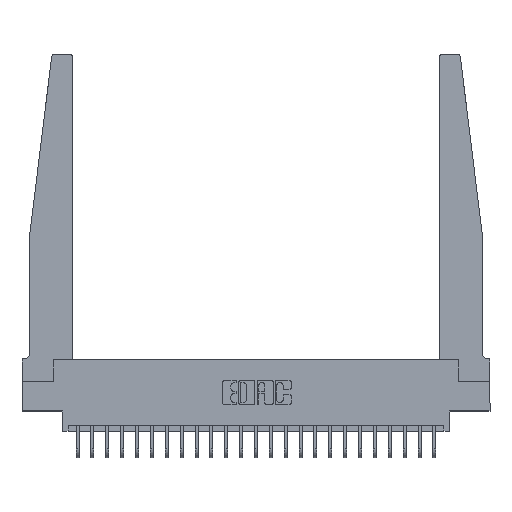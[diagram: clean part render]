
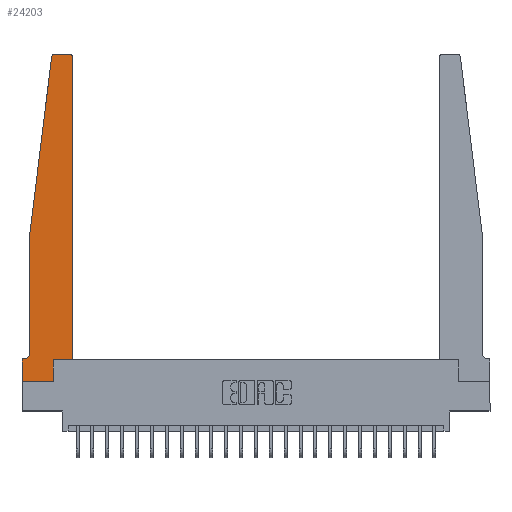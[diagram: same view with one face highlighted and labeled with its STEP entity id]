
A CAD part, top view. The second image highlights one B-rep face of the part: STEP entity #24203.
In plain terms, the highlighted planar face has unit normal (0, 0, 1).
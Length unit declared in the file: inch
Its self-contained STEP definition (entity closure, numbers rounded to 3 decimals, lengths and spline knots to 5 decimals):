
#118 = LINE ( 'NONE', #17235, #22158 ) ;
#379 = EDGE_CURVE ( 'NONE', #5622, #12134, #1191, .T. ) ;
#877 = CARTESIAN_POINT ( 'NONE',  ( 0.065, 1.25, 0.37 ) ) ;
#941 = DIRECTION ( 'NONE',  ( 0., 1., 0. ) ) ;
#982 = ORIENTED_EDGE ( 'NONE', *, *, #8658, .T. ) ;
#1095 = EDGE_CURVE ( 'NONE', #8625, #15028, #19978, .T. ) ;
#1191 = CIRCLE ( 'NONE', #22807, 0.05 ) ;
#1238 = EDGE_LOOP ( 'NONE', ( #15149, #24596, #18126, #21633, #3442, #11357, #982, #8872, #19196, #20219, #20866, #9613 ) ) ;
#1828 = DIRECTION ( 'NONE',  ( 0., 0., -1. ) ) ;
#1925 = EDGE_CURVE ( 'NONE', #3250, #15657, #21378, .T. ) ;
#2043 = AXIS2_PLACEMENT_3D ( 'NONE', #4962, #18669, #22398 ) ;
#2256 = CARTESIAN_POINT ( 'NONE',  ( 0.25, 2.75, 0.37 ) ) ;
#2316 = DIRECTION ( 'NONE',  ( 1., 0., 0. ) ) ;
#2457 = DIRECTION ( 'NONE',  ( 1., 0., 0. ) ) ;
#2636 = EDGE_CURVE ( 'NONE', #15657, #2741, #11754, .T. ) ;
#2741 = VERTEX_POINT ( 'NONE', #22405 ) ;
#2811 = DIRECTION ( 'NONE',  ( 0., 0., 1. ) ) ;
#3103 = DIRECTION ( 'NONE',  ( 0., 1., 0. ) ) ;
#3250 = VERTEX_POINT ( 'NONE', #22775 ) ;
#3420 = DIRECTION ( 'NONE',  ( 1., 0., 0. ) ) ;
#3442 = ORIENTED_EDGE ( 'NONE', *, *, #379, .T. ) ;
#3671 = VERTEX_POINT ( 'NONE', #18978 ) ;
#3898 = DIRECTION ( 'NONE',  ( 0., -1., 0. ) ) ;
#4397 = CARTESIAN_POINT ( 'NONE',  ( 0.2605, 0.18, 0.37 ) ) ;
#4804 = VERTEX_POINT ( 'NONE', #24318 ) ;
#4962 = CARTESIAN_POINT ( 'NONE',  ( 0.395, 2.72, 0.37 ) ) ;
#5622 = VERTEX_POINT ( 'NONE', #9046 ) ;
#5848 = CARTESIAN_POINT ( 'NONE',  ( 0.24675, 2.72367, 0.37 ) ) ;
#5886 = CIRCLE ( 'NONE', #2043, 0.03 ) ;
#6348 = LINE ( 'NONE', #14084, #6636 ) ;
#6408 = CARTESIAN_POINT ( 'NONE',  ( 0., 0., 0.37 ) ) ;
#6636 = VECTOR ( 'NONE', #2316, 39.37008 ) ;
#6832 = PLANE ( 'NONE',  #20390 ) ;
#6907 = LINE ( 'NONE', #16266, #21866 ) ;
#7253 = CARTESIAN_POINT ( 'NONE',  ( 0.425, 0.18, 0.37 ) ) ;
#7328 = CARTESIAN_POINT ( 'NONE',  ( 0.425, 0.18, 0.37 ) ) ;
#7578 = DIRECTION ( 'NONE',  ( 1., 0., 0. ) ) ;
#8194 = DIRECTION ( 'NONE',  ( -1., 0., 0. ) ) ;
#8625 = VERTEX_POINT ( 'NONE', #23300 ) ;
#8658 = EDGE_CURVE ( 'NONE', #3671, #12701, #13983, .T. ) ;
#8826 = EDGE_CURVE ( 'NONE', #14636, #24458, #6907, .T. ) ;
#8872 = ORIENTED_EDGE ( 'NONE', *, *, #17418, .T. ) ;
#9046 = CARTESIAN_POINT ( 'NONE',  ( 0.065, 0.2375, 0.37 ) ) ;
#9503 = EDGE_CURVE ( 'NONE', #24458, #5622, #13609, .T. ) ;
#9613 = ORIENTED_EDGE ( 'NONE', *, *, #15173, .T. ) ;
#9678 = EDGE_CURVE ( 'NONE', #4804, #3250, #17553, .T. ) ;
#10190 = DIRECTION ( 'NONE',  ( 0., -1., 0. ) ) ;
#10811 = CIRCLE ( 'NONE', #14279, 0.03 ) ;
#10902 = FACE_OUTER_BOUND ( 'NONE', #1238, .T. ) ;
#11131 = VECTOR ( 'NONE', #3103, 39.37008 ) ;
#11153 = DIRECTION ( 'NONE',  ( -0.122, -0.992, 0. ) ) ;
#11357 = ORIENTED_EDGE ( 'NONE', *, *, #13931, .T. ) ;
#11508 = CARTESIAN_POINT ( 'NONE',  ( 0.27653, 2.75, 0.37 ) ) ;
#11754 = LINE ( 'NONE', #7253, #11131 ) ;
#12134 = VERTEX_POINT ( 'NONE', #16820 ) ;
#12701 = VERTEX_POINT ( 'NONE', #13743 ) ;
#13284 = DIRECTION ( 'NONE',  ( -1., 0., 0. ) ) ;
#13378 = VECTOR ( 'NONE', #3898, 39.37008 ) ;
#13400 = DIRECTION ( 'NONE',  ( 0., 0., 1. ) ) ;
#13609 = LINE ( 'NONE', #17940, #18164 ) ;
#13743 = CARTESIAN_POINT ( 'NONE',  ( 0., 0., 0.37 ) ) ;
#13931 = EDGE_CURVE ( 'NONE', #12134, #3671, #118, .T. ) ;
#13983 = LINE ( 'NONE', #6408, #13378 ) ;
#14084 = CARTESIAN_POINT ( 'NONE',  ( 0., 0., 0.37 ) ) ;
#14279 = AXIS2_PLACEMENT_3D ( 'NONE', #24258, #2811, #2457 ) ;
#14636 = VERTEX_POINT ( 'NONE', #5848 ) ;
#15028 = VERTEX_POINT ( 'NONE', #11508 ) ;
#15034 = CARTESIAN_POINT ( 'NONE',  ( 0.425, 0.18, 0.37 ) ) ;
#15149 = ORIENTED_EDGE ( 'NONE', *, *, #1095, .T. ) ;
#15173 = EDGE_CURVE ( 'NONE', #2741, #8625, #5886, .T. ) ;
#15657 = VERTEX_POINT ( 'NONE', #15034 ) ;
#15727 = VECTOR ( 'NONE', #8194, 39.37008 ) ;
#16266 = CARTESIAN_POINT ( 'NONE',  ( 0.065, 1.25, 0.37 ) ) ;
#16347 = VECTOR ( 'NONE', #941, 39.37008 ) ;
#16820 = CARTESIAN_POINT ( 'NONE',  ( 0.015, 0.1875, 0.37 ) ) ;
#17235 = CARTESIAN_POINT ( 'NONE',  ( 0.065, 0.1875, 0.37 ) ) ;
#17418 = EDGE_CURVE ( 'NONE', #12701, #4804, #6348, .T. ) ;
#17553 = LINE ( 'NONE', #4397, #16347 ) ;
#17940 = CARTESIAN_POINT ( 'NONE',  ( 0.065, 1.25, 0.37 ) ) ;
#18126 = ORIENTED_EDGE ( 'NONE', *, *, #8826, .T. ) ;
#18164 = VECTOR ( 'NONE', #10190, 39.37008 ) ;
#18353 = VECTOR ( 'NONE', #7578, 39.37008 ) ;
#18669 = DIRECTION ( 'NONE',  ( 0., 0., 1. ) ) ;
#18978 = CARTESIAN_POINT ( 'NONE',  ( 0., 0.1875, 0.37 ) ) ;
#19196 = ORIENTED_EDGE ( 'NONE', *, *, #9678, .T. ) ;
#19978 = LINE ( 'NONE', #2256, #15727 ) ;
#20181 = EDGE_CURVE ( 'NONE', #15028, #14636, #10811, .T. ) ;
#20219 = ORIENTED_EDGE ( 'NONE', *, *, #1925, .T. ) ;
#20390 = AXIS2_PLACEMENT_3D ( 'NONE', #25040, #13400, #3420 ) ;
#20866 = ORIENTED_EDGE ( 'NONE', *, *, #2636, .T. ) ;
#21378 = LINE ( 'NONE', #7328, #18353 ) ;
#21633 = ORIENTED_EDGE ( 'NONE', *, *, #9503, .T. ) ;
#21866 = VECTOR ( 'NONE', #11153, 39.37008 ) ;
#22158 = VECTOR ( 'NONE', #23093, 39.37008 ) ;
#22398 = DIRECTION ( 'NONE',  ( 1., 0., 0. ) ) ;
#22405 = CARTESIAN_POINT ( 'NONE',  ( 0.425, 2.72, 0.37 ) ) ;
#22775 = CARTESIAN_POINT ( 'NONE',  ( 0.2605, 0.18, 0.37 ) ) ;
#22807 = AXIS2_PLACEMENT_3D ( 'NONE', #24917, #1828, #13284 ) ;
#23093 = DIRECTION ( 'NONE',  ( -1., 0., 0. ) ) ;
#23300 = CARTESIAN_POINT ( 'NONE',  ( 0.395, 2.75, 0.37 ) ) ;
#24203 = ADVANCED_FACE ( 'NONE', ( #10902 ), #6832, .T. ) ;
#24258 = CARTESIAN_POINT ( 'NONE',  ( 0.27653, 2.72, 0.37 ) ) ;
#24318 = CARTESIAN_POINT ( 'NONE',  ( 0.2605, 0., 0.37 ) ) ;
#24458 = VERTEX_POINT ( 'NONE', #877 ) ;
#24596 = ORIENTED_EDGE ( 'NONE', *, *, #20181, .T. ) ;
#24917 = CARTESIAN_POINT ( 'NONE',  ( 0.015, 0.2375, 0.37 ) ) ;
#25040 = CARTESIAN_POINT ( 'NONE',  ( 0., 0.1875, 0.37 ) ) ;
